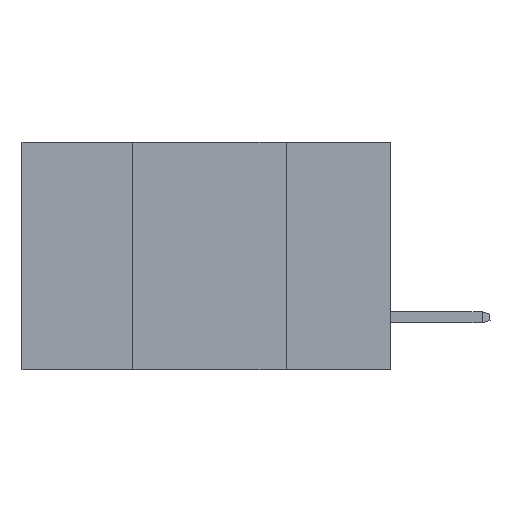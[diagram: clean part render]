
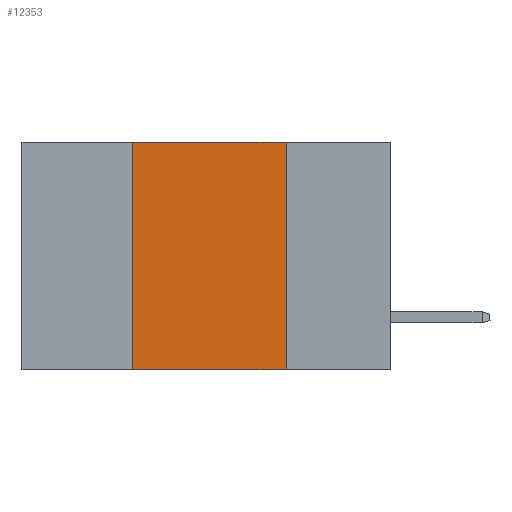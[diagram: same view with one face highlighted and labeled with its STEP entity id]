
A CAD part, left-side view. The second image highlights one B-rep face of the part: STEP entity #12353.
In plain terms, the highlighted planar face has unit normal (-1, 0, 0).
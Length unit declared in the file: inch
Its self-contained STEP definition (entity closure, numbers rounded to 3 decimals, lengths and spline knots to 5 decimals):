
#529 = VERTEX_POINT ( 'NONE', #5161 ) ;
#2770 = VERTEX_POINT ( 'NONE', #23355 ) ;
#3424 = CARTESIAN_POINT ( 'NONE',  ( 0., 0.6, 0. ) ) ;
#5127 = CARTESIAN_POINT ( 'NONE',  ( 0., 0.6, -0.37 ) ) ;
#5161 = CARTESIAN_POINT ( 'NONE',  ( 0., 0.17, -0.37 ) ) ;
#5266 = FACE_OUTER_BOUND ( 'NONE', #6555, .T. ) ;
#5526 = ORIENTED_EDGE ( 'NONE', *, *, #18524, .F. ) ;
#5865 = CARTESIAN_POINT ( 'NONE',  ( 0., 0.42, 0. ) ) ;
#6555 = EDGE_LOOP ( 'NONE', ( #15658, #5526, #22227, #7426 ) ) ;
#7171 = DIRECTION ( 'NONE',  ( 0., -1., 0. ) ) ;
#7426 = ORIENTED_EDGE ( 'NONE', *, *, #12212, .T. ) ;
#7819 = VECTOR ( 'NONE', #7171, 39.37008 ) ;
#8128 = VECTOR ( 'NONE', #19551, 39.37008 ) ;
#8533 = CARTESIAN_POINT ( 'NONE',  ( 0., 0.17, 0. ) ) ;
#9219 = CARTESIAN_POINT ( 'NONE',  ( 0., 0.17, 0. ) ) ;
#10693 = EDGE_CURVE ( 'NONE', #2770, #11809, #13591, .T. ) ;
#11570 = DIRECTION ( 'NONE',  ( 1., 0., 0. ) ) ;
#11809 = VERTEX_POINT ( 'NONE', #5865 ) ;
#12212 = EDGE_CURVE ( 'NONE', #2770, #529, #23890, .T. ) ;
#12241 = VERTEX_POINT ( 'NONE', #9219 ) ;
#12353 = ADVANCED_FACE ( 'NONE', ( #5266 ), #21628, .F. ) ;
#12549 = DIRECTION ( 'NONE',  ( 0., 0., -1. ) ) ;
#13272 = EDGE_CURVE ( 'NONE', #12241, #529, #14089, .T. ) ;
#13500 = LINE ( 'NONE', #3424, #8128 ) ;
#13591 = LINE ( 'NONE', #20212, #23656 ) ;
#14089 = LINE ( 'NONE', #8533, #24132 ) ;
#15342 = AXIS2_PLACEMENT_3D ( 'NONE', #23632, #11570, #25645 ) ;
#15658 = ORIENTED_EDGE ( 'NONE', *, *, #13272, .F. ) ;
#16186 = DIRECTION ( 'NONE',  ( 0., 0., 1. ) ) ;
#18524 = EDGE_CURVE ( 'NONE', #11809, #12241, #13500, .T. ) ;
#19551 = DIRECTION ( 'NONE',  ( 0., -1., 0. ) ) ;
#20212 = CARTESIAN_POINT ( 'NONE',  ( 0., 0.42, 0. ) ) ;
#21628 = PLANE ( 'NONE',  #15342 ) ;
#22227 = ORIENTED_EDGE ( 'NONE', *, *, #10693, .F. ) ;
#23355 = CARTESIAN_POINT ( 'NONE',  ( 0., 0.42, -0.37 ) ) ;
#23632 = CARTESIAN_POINT ( 'NONE',  ( 0., 0.6, 0. ) ) ;
#23656 = VECTOR ( 'NONE', #16186, 39.37008 ) ;
#23890 = LINE ( 'NONE', #5127, #7819 ) ;
#24132 = VECTOR ( 'NONE', #12549, 39.37008 ) ;
#25645 = DIRECTION ( 'NONE',  ( 0., 0., -1. ) ) ;
